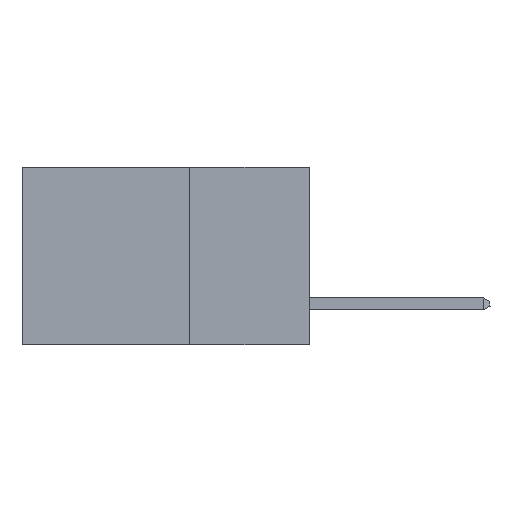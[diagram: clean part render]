
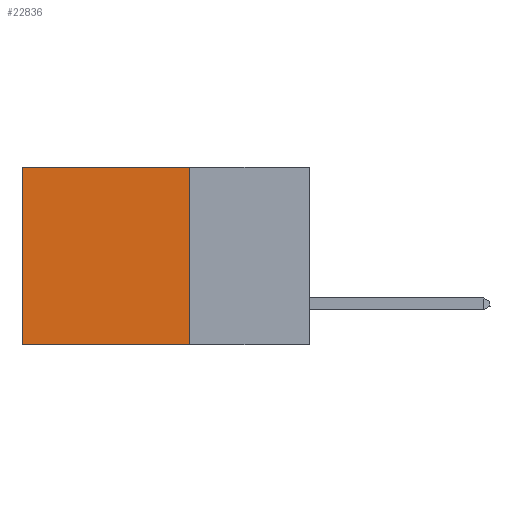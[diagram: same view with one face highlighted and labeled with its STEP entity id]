
A CAD part, left-side view. The second image highlights one B-rep face of the part: STEP entity #22836.
In plain terms, the highlighted planar face has unit normal (-1, 0, 0).
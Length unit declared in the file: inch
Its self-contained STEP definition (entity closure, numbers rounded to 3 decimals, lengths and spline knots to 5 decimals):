
#269 = VERTEX_POINT ( 'NONE', #32307 ) ;
#1198 = VECTOR ( 'NONE', #25490, 39.37008 ) ;
#3648 = VERTEX_POINT ( 'NONE', #26945 ) ;
#4199 = LINE ( 'NONE', #7351, #22250 ) ;
#5446 = DIRECTION ( 'NONE',  ( 0., 0., -1. ) ) ;
#5521 = VECTOR ( 'NONE', #25082, 39.37008 ) ;
#7351 = CARTESIAN_POINT ( 'NONE',  ( 0.2875, 0.25, 0. ) ) ;
#7817 = EDGE_CURVE ( 'NONE', #34661, #3648, #28530, .T. ) ;
#10413 = VECTOR ( 'NONE', #27144, 39.37008 ) ;
#11408 = PLANE ( 'NONE',  #26946 ) ;
#12240 = LINE ( 'NONE', #27419, #10413 ) ;
#13386 = EDGE_CURVE ( 'NONE', #34661, #269, #4199, .T. ) ;
#18840 = CARTESIAN_POINT ( 'NONE',  ( 0.2875, 0.25, -0.37 ) ) ;
#21988 = EDGE_CURVE ( 'NONE', #269, #26693, #12240, .T. ) ;
#22250 = VECTOR ( 'NONE', #30714, 39.37008 ) ;
#22836 = ADVANCED_FACE ( 'NONE', ( #23525 ), #11408, .F. ) ;
#23105 = LINE ( 'NONE', #18840, #5521 ) ;
#23525 = FACE_OUTER_BOUND ( 'NONE', #30394, .T. ) ;
#25082 = DIRECTION ( 'NONE',  ( 0., 1., 0. ) ) ;
#25490 = DIRECTION ( 'NONE',  ( 0., 0., -1. ) ) ;
#25947 = CARTESIAN_POINT ( 'NONE',  ( 0.2875, 0.25, 0. ) ) ;
#26693 = VERTEX_POINT ( 'NONE', #36598 ) ;
#26945 = CARTESIAN_POINT ( 'NONE',  ( 0.2875, 0.25, -0.37 ) ) ;
#26946 = AXIS2_PLACEMENT_3D ( 'NONE', #32148, #28916, #5446 ) ;
#27144 = DIRECTION ( 'NONE',  ( 0., 0., -1. ) ) ;
#27419 = CARTESIAN_POINT ( 'NONE',  ( 0.2875, 0.6, 0. ) ) ;
#27900 = EDGE_CURVE ( 'NONE', #3648, #26693, #23105, .T. ) ;
#28530 = LINE ( 'NONE', #31851, #1198 ) ;
#28916 = DIRECTION ( 'NONE',  ( 1., 0., 0. ) ) ;
#30394 = EDGE_LOOP ( 'NONE', ( #37394, #38372, #38070, #37368 ) ) ;
#30714 = DIRECTION ( 'NONE',  ( 0., 1., 0. ) ) ;
#31851 = CARTESIAN_POINT ( 'NONE',  ( 0.2875, 0.25, 0. ) ) ;
#32148 = CARTESIAN_POINT ( 'NONE',  ( 0.2875, 0.25, 0. ) ) ;
#32307 = CARTESIAN_POINT ( 'NONE',  ( 0.2875, 0.6, 0. ) ) ;
#34661 = VERTEX_POINT ( 'NONE', #25947 ) ;
#36598 = CARTESIAN_POINT ( 'NONE',  ( 0.2875, 0.6, -0.37 ) ) ;
#37368 = ORIENTED_EDGE ( 'NONE', *, *, #13386, .T. ) ;
#37394 = ORIENTED_EDGE ( 'NONE', *, *, #21988, .T. ) ;
#38070 = ORIENTED_EDGE ( 'NONE', *, *, #7817, .F. ) ;
#38372 = ORIENTED_EDGE ( 'NONE', *, *, #27900, .F. ) ;
